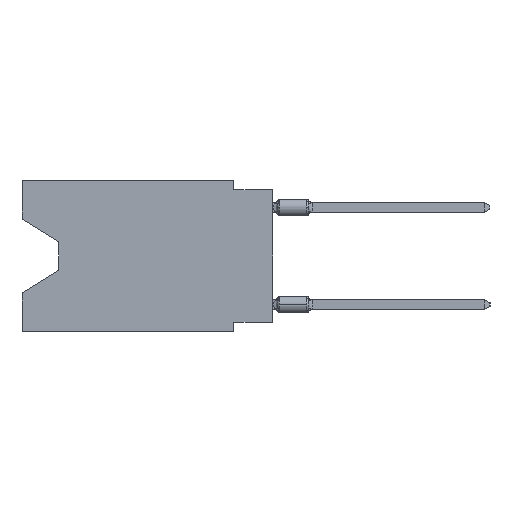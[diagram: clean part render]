
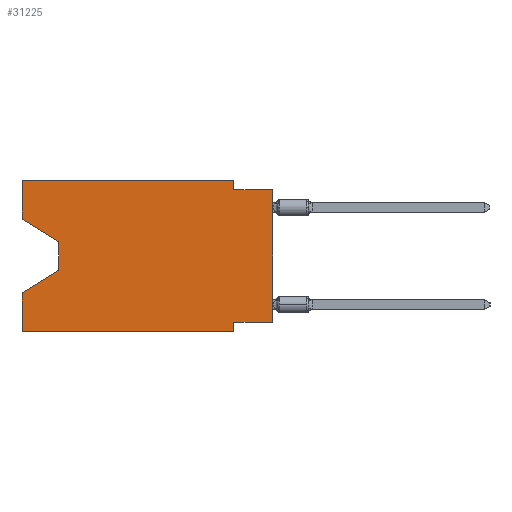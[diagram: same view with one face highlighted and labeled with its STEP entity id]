
A CAD part, left-side view. The second image highlights one B-rep face of the part: STEP entity #31225.
In plain terms, the highlighted planar face has unit normal (-1, 0, 0).
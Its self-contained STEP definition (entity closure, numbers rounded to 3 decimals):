
#2246 = PLANE ( 'NONE',  #37102 ) ;
#2681 = EDGE_CURVE ( 'NONE', #26025, #26481, #31730, .T. ) ;
#2878 = CARTESIAN_POINT ( 'NONE',  ( 0., 16.383, -2.546 ) ) ;
#3481 = ORIENTED_EDGE ( 'NONE', *, *, #4058, .T. ) ;
#3569 = ORIENTED_EDGE ( 'NONE', *, *, #34226, .T. ) ;
#4058 = EDGE_CURVE ( 'NONE', #34482, #30354, #17245, .T. ) ;
#4243 = LINE ( 'NONE', #37346, #7267 ) ;
#4882 = CARTESIAN_POINT ( 'NONE',  ( 0., 0., -9.271 ) ) ;
#4922 = ORIENTED_EDGE ( 'NONE', *, *, #31164, .F. ) ;
#5002 = DIRECTION ( 'NONE',  ( 0., 0., -1. ) ) ;
#5030 = LINE ( 'NONE', #32510, #32622 ) ;
#5185 = DIRECTION ( 'NONE',  ( 0., -1., 0. ) ) ;
#5249 = LINE ( 'NONE', #23295, #24443 ) ;
#5722 = VECTOR ( 'NONE', #28910, 1000. ) ;
#6261 = VECTOR ( 'NONE', #11067, 1000. ) ;
#6619 = EDGE_CURVE ( 'NONE', #20998, #34482, #23909, .T. ) ;
#7003 = EDGE_CURVE ( 'NONE', #20998, #36816, #8986, .T. ) ;
#7267 = VECTOR ( 'NONE', #15894, 1000. ) ;
#7648 = FACE_OUTER_BOUND ( 'NONE', #16832, .T. ) ;
#8049 = DIRECTION ( 'NONE',  ( 0., 0., -1. ) ) ;
#8199 = DIRECTION ( 'NONE',  ( 0., -1., 0. ) ) ;
#8986 = LINE ( 'NONE', #18017, #39282 ) ;
#9758 = VECTOR ( 'NONE', #5002, 1000. ) ;
#9872 = CARTESIAN_POINT ( 'NONE',  ( 0., 16.383, -2.546 ) ) ;
#10474 = DIRECTION ( 'NONE',  ( 1., 0., 0. ) ) ;
#11067 = DIRECTION ( 'NONE',  ( 0., 1., 0. ) ) ;
#11226 = LINE ( 'NONE', #23436, #11537 ) ;
#11370 = VERTEX_POINT ( 'NONE', #14170 ) ;
#11537 = VECTOR ( 'NONE', #8199, 1000. ) ;
#11796 = VERTEX_POINT ( 'NONE', #4882 ) ;
#11877 = CARTESIAN_POINT ( 'NONE',  ( 0., 16.383, -9.906 ) ) ;
#12001 = DIRECTION ( 'NONE',  ( 0., 0., 1. ) ) ;
#13568 = ORIENTED_EDGE ( 'NONE', *, *, #7003, .F. ) ;
#14146 = VECTOR ( 'NONE', #32872, 1000. ) ;
#14170 = CARTESIAN_POINT ( 'NONE',  ( 0., 2.54, 0. ) ) ;
#14278 = LINE ( 'NONE', #32706, #34121 ) ;
#14360 = ORIENTED_EDGE ( 'NONE', *, *, #27211, .F. ) ;
#14743 = EDGE_CURVE ( 'NONE', #11796, #33328, #17487, .T. ) ;
#15894 = DIRECTION ( 'NONE',  ( 0., -1., 0. ) ) ;
#16181 = ORIENTED_EDGE ( 'NONE', *, *, #33023, .T. ) ;
#16687 = DIRECTION ( 'NONE',  ( 0., 0., -1. ) ) ;
#16725 = ORIENTED_EDGE ( 'NONE', *, *, #30275, .T. ) ;
#16832 = EDGE_LOOP ( 'NONE', ( #36165, #3481, #16181, #29607, #16725, #4922, #26459, #3569, #14360, #37777, #39620, #13568 ) ) ;
#17245 = LINE ( 'NONE', #29475, #9758 ) ;
#17487 = LINE ( 'NONE', #27291, #6261 ) ;
#18017 = CARTESIAN_POINT ( 'NONE',  ( 0., 16.383, 0. ) ) ;
#18041 = CARTESIAN_POINT ( 'NONE',  ( 0., 13.97, -5.893 ) ) ;
#19694 = CARTESIAN_POINT ( 'NONE',  ( 0., 16.383, 0. ) ) ;
#20634 = LINE ( 'NONE', #18041, #14146 ) ;
#20998 = VERTEX_POINT ( 'NONE', #9872 ) ;
#21023 = CARTESIAN_POINT ( 'NONE',  ( 0., 0., -0.635 ) ) ;
#21591 = VECTOR ( 'NONE', #5185, 1000. ) ;
#22150 = VERTEX_POINT ( 'NONE', #39558 ) ;
#22236 = EDGE_CURVE ( 'NONE', #36816, #11370, #4243, .T. ) ;
#23228 = CARTESIAN_POINT ( 'NONE',  ( 0., 2.54, -0.635 ) ) ;
#23270 = VECTOR ( 'NONE', #24303, 1000. ) ;
#23295 = CARTESIAN_POINT ( 'NONE',  ( 0., 0., 0. ) ) ;
#23436 = CARTESIAN_POINT ( 'NONE',  ( 0., 16.383, -9.906 ) ) ;
#23582 = CARTESIAN_POINT ( 'NONE',  ( 0., 13.97, -4.013 ) ) ;
#23889 = DIRECTION ( 'NONE',  ( 0., 0., 1. ) ) ;
#23909 = LINE ( 'NONE', #2878, #23270 ) ;
#24141 = CARTESIAN_POINT ( 'NONE',  ( 0., 16.383, -7.36 ) ) ;
#24303 = DIRECTION ( 'NONE',  ( 0., -0.855, -0.519 ) ) ;
#24443 = VECTOR ( 'NONE', #23889, 1000. ) ;
#26025 = VERTEX_POINT ( 'NONE', #11877 ) ;
#26459 = ORIENTED_EDGE ( 'NONE', *, *, #14743, .F. ) ;
#26481 = VERTEX_POINT ( 'NONE', #24141 ) ;
#26686 = CARTESIAN_POINT ( 'NONE',  ( 0., 16.383, 0. ) ) ;
#26690 = DIRECTION ( 'NONE',  ( 0., 0., -1. ) ) ;
#27138 = VERTEX_POINT ( 'NONE', #23228 ) ;
#27211 = EDGE_CURVE ( 'NONE', #27138, #32364, #36273, .T. ) ;
#27291 = CARTESIAN_POINT ( 'NONE',  ( 0., 0., -9.271 ) ) ;
#28910 = DIRECTION ( 'NONE',  ( 0., 0., 1. ) ) ;
#29475 = CARTESIAN_POINT ( 'NONE',  ( 0., 13.97, -4.013 ) ) ;
#29607 = ORIENTED_EDGE ( 'NONE', *, *, #2681, .F. ) ;
#30275 = EDGE_CURVE ( 'NONE', #26025, #22150, #11226, .T. ) ;
#30354 = VERTEX_POINT ( 'NONE', #34069 ) ;
#30815 = CARTESIAN_POINT ( 'NONE',  ( 0., 0., -0.635 ) ) ;
#31164 = EDGE_CURVE ( 'NONE', #33328, #22150, #5030, .T. ) ;
#31225 = ADVANCED_FACE ( 'NONE', ( #7648 ), #2246, .F. ) ;
#31730 = LINE ( 'NONE', #19694, #5722 ) ;
#32364 = VERTEX_POINT ( 'NONE', #30815 ) ;
#32510 = CARTESIAN_POINT ( 'NONE',  ( 0., 2.54, -9.906 ) ) ;
#32622 = VECTOR ( 'NONE', #8049, 1000. ) ;
#32706 = CARTESIAN_POINT ( 'NONE',  ( 0., 2.54, 0. ) ) ;
#32823 = CARTESIAN_POINT ( 'NONE',  ( 0., 2.54, -9.271 ) ) ;
#32872 = DIRECTION ( 'NONE',  ( 0., 0.855, -0.519 ) ) ;
#33023 = EDGE_CURVE ( 'NONE', #30354, #26481, #20634, .T. ) ;
#33328 = VERTEX_POINT ( 'NONE', #32823 ) ;
#34069 = CARTESIAN_POINT ( 'NONE',  ( 0., 13.97, -5.893 ) ) ;
#34121 = VECTOR ( 'NONE', #26690, 1000. ) ;
#34226 = EDGE_CURVE ( 'NONE', #11796, #32364, #5249, .T. ) ;
#34482 = VERTEX_POINT ( 'NONE', #23582 ) ;
#34842 = CARTESIAN_POINT ( 'NONE',  ( 0., 16.383, 0. ) ) ;
#34981 = EDGE_CURVE ( 'NONE', #11370, #27138, #14278, .T. ) ;
#36165 = ORIENTED_EDGE ( 'NONE', *, *, #6619, .T. ) ;
#36273 = LINE ( 'NONE', #21023, #21591 ) ;
#36816 = VERTEX_POINT ( 'NONE', #34842 ) ;
#37102 = AXIS2_PLACEMENT_3D ( 'NONE', #26686, #10474, #16687 ) ;
#37346 = CARTESIAN_POINT ( 'NONE',  ( 0., 16.383, 0. ) ) ;
#37777 = ORIENTED_EDGE ( 'NONE', *, *, #34981, .F. ) ;
#39282 = VECTOR ( 'NONE', #12001, 1000. ) ;
#39558 = CARTESIAN_POINT ( 'NONE',  ( 0., 2.54, -9.906 ) ) ;
#39620 = ORIENTED_EDGE ( 'NONE', *, *, #22236, .F. ) ;
